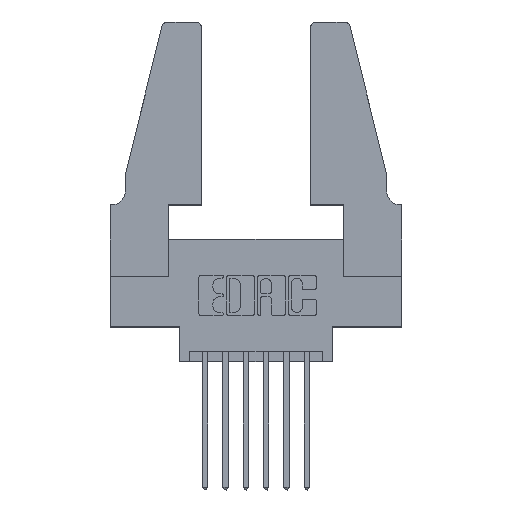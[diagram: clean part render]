
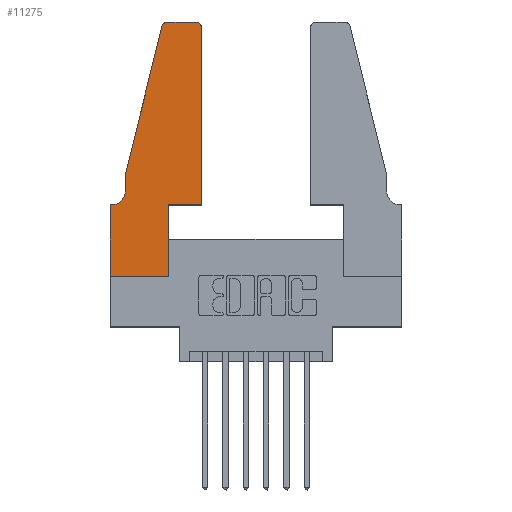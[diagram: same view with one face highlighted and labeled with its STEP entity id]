
A CAD part, top view. The second image highlights one B-rep face of the part: STEP entity #11275.
In plain terms, the highlighted planar face has unit normal (0, 0, 1).
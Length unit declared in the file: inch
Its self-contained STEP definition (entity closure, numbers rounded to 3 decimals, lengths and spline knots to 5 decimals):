
#125 = DIRECTION ( 'NONE',  ( 0., 0., 1. ) ) ;
#159 = VECTOR ( 'NONE', #10618, 39.37008 ) ;
#268 = CARTESIAN_POINT ( 'NONE',  ( 0.0755, 0.42, 0.37 ) ) ;
#296 = EDGE_CURVE ( 'NONE', #6114, #10409, #2777, .T. ) ;
#337 = ORIENTED_EDGE ( 'NONE', *, *, #775, .T. ) ;
#411 = LINE ( 'NONE', #1375, #7458 ) ;
#775 = EDGE_CURVE ( 'NONE', #4397, #8239, #9487, .T. ) ;
#880 = DIRECTION ( 'NONE',  ( 0., 1., 0. ) ) ;
#883 = AXIS2_PLACEMENT_3D ( 'NONE', #7408, #7366, #7343 ) ;
#1273 = AXIS2_PLACEMENT_3D ( 'NONE', #11120, #125, #6555 ) ;
#1285 = CARTESIAN_POINT ( 'NONE',  ( 0.4205, 1.22, 0.37 ) ) ;
#1375 = CARTESIAN_POINT ( 'NONE',  ( 0., 0., 0.37 ) ) ;
#1413 = CARTESIAN_POINT ( 'NONE',  ( 0.2865, 0., 0.37 ) ) ;
#1421 = DIRECTION ( 'NONE',  ( 1., 0., 0. ) ) ;
#1423 = DIRECTION ( 'NONE',  ( 0., 0., 1. ) ) ;
#1578 = DIRECTION ( 'NONE',  ( 0., -1., 0. ) ) ;
#1852 = VECTOR ( 'NONE', #880, 39.37008 ) ;
#2262 = CARTESIAN_POINT ( 'NONE',  ( 0.0755, 0.5, 0.37 ) ) ;
#2398 = EDGE_CURVE ( 'NONE', #9714, #2698, #7152, .T. ) ;
#2428 = ORIENTED_EDGE ( 'NONE', *, *, #6480, .T. ) ;
#2453 = AXIS2_PLACEMENT_3D ( 'NONE', #1285, #1423, #1421 ) ;
#2611 = CARTESIAN_POINT ( 'NONE',  ( 0.4505, 0.35, 0.37 ) ) ;
#2621 = LINE ( 'NONE', #8940, #8468 ) ;
#2698 = VERTEX_POINT ( 'NONE', #5643 ) ;
#2777 = LINE ( 'NONE', #4237, #4912 ) ;
#2834 = VERTEX_POINT ( 'NONE', #1413 ) ;
#2929 = LINE ( 'NONE', #4214, #159 ) ;
#2939 = ORIENTED_EDGE ( 'NONE', *, *, #296, .T. ) ;
#3159 = VERTEX_POINT ( 'NONE', #5453 ) ;
#3392 = ORIENTED_EDGE ( 'NONE', *, *, #8970, .T. ) ;
#3444 = DIRECTION ( 'NONE',  ( 1., 0., 0. ) ) ;
#3643 = EDGE_CURVE ( 'NONE', #3159, #10041, #5273, .T. ) ;
#4009 = DIRECTION ( 'NONE',  ( -0.239, -0.971, 0. ) ) ;
#4214 = CARTESIAN_POINT ( 'NONE',  ( 0., 0., 0.37 ) ) ;
#4237 = CARTESIAN_POINT ( 'NONE',  ( 0.4505, 0.35, 0.37 ) ) ;
#4397 = VERTEX_POINT ( 'NONE', #268 ) ;
#4485 = EDGE_CURVE ( 'NONE', #2834, #6114, #5528, .T. ) ;
#4746 = ORIENTED_EDGE ( 'NONE', *, *, #5229, .T. ) ;
#4912 = VECTOR ( 'NONE', #3444, 39.37008 ) ;
#5229 = EDGE_CURVE ( 'NONE', #9911, #2834, #2929, .T. ) ;
#5273 = CIRCLE ( 'NONE', #883, 0.03 ) ;
#5312 = FACE_OUTER_BOUND ( 'NONE', #9734, .T. ) ;
#5453 = CARTESIAN_POINT ( 'NONE',  ( 0.284, 1.25, 0.37 ) ) ;
#5528 = LINE ( 'NONE', #9591, #10395 ) ;
#5643 = CARTESIAN_POINT ( 'NONE',  ( 0.4205, 1.25, 0.37 ) ) ;
#5646 = PLANE ( 'NONE',  #1273 ) ;
#5889 = CARTESIAN_POINT ( 'NONE',  ( 0., 0., 0.37 ) ) ;
#5905 = LINE ( 'NONE', #9854, #10490 ) ;
#5943 = DIRECTION ( 'NONE',  ( 0., -1., 0. ) ) ;
#6023 = VECTOR ( 'NONE', #4009, 39.37008 ) ;
#6092 = CARTESIAN_POINT ( 'NONE',  ( 0.25487, 1.22718, 0.37 ) ) ;
#6114 = VERTEX_POINT ( 'NONE', #9240 ) ;
#6282 = ORIENTED_EDGE ( 'NONE', *, *, #7153, .T. ) ;
#6480 = EDGE_CURVE ( 'NONE', #8020, #4397, #5905, .T. ) ;
#6555 = DIRECTION ( 'NONE',  ( 1., 0., 0. ) ) ;
#6924 = CARTESIAN_POINT ( 'NONE',  ( 0., 0.35, 0.37 ) ) ;
#6997 = LINE ( 'NONE', #10938, #1852 ) ;
#7152 = CIRCLE ( 'NONE', #2453, 0.03 ) ;
#7153 = EDGE_CURVE ( 'NONE', #2698, #3159, #2621, .T. ) ;
#7343 = DIRECTION ( 'NONE',  ( 1., 0., 0. ) ) ;
#7366 = DIRECTION ( 'NONE',  ( 0., 0., 1. ) ) ;
#7408 = CARTESIAN_POINT ( 'NONE',  ( 0.284, 1.22, 0.37 ) ) ;
#7458 = VECTOR ( 'NONE', #5943, 39.37008 ) ;
#7779 = DIRECTION ( 'NONE',  ( 0., 1., 0. ) ) ;
#8020 = VERTEX_POINT ( 'NONE', #2262 ) ;
#8239 = VERTEX_POINT ( 'NONE', #10840 ) ;
#8261 = CARTESIAN_POINT ( 'NONE',  ( 0.0755, 0.35, 0.37 ) ) ;
#8319 = VECTOR ( 'NONE', #11016, 39.37008 ) ;
#8453 = LINE ( 'NONE', #11273, #6023 ) ;
#8468 = VECTOR ( 'NONE', #11626, 39.37008 ) ;
#8940 = CARTESIAN_POINT ( 'NONE',  ( 0.2605, 1.25, 0.37 ) ) ;
#8970 = EDGE_CURVE ( 'NONE', #10409, #9714, #6997, .T. ) ;
#9240 = CARTESIAN_POINT ( 'NONE',  ( 0.2865, 0.35, 0.37 ) ) ;
#9294 = CARTESIAN_POINT ( 'NONE',  ( 0.4505, 1.22, 0.37 ) ) ;
#9326 = AXIS2_PLACEMENT_3D ( 'NONE', #10388, #10371, #10266 ) ;
#9349 = VERTEX_POINT ( 'NONE', #6924 ) ;
#9384 = ORIENTED_EDGE ( 'NONE', *, *, #3643, .T. ) ;
#9487 = CIRCLE ( 'NONE', #9326, 0.07 ) ;
#9591 = CARTESIAN_POINT ( 'NONE',  ( 0.2865, 0.35, 0.37 ) ) ;
#9714 = VERTEX_POINT ( 'NONE', #9294 ) ;
#9734 = EDGE_LOOP ( 'NONE', ( #6282, #9384, #10839, #2428, #337, #10258, #10507, #4746, #9831, #2939, #3392, #11041 ) ) ;
#9831 = ORIENTED_EDGE ( 'NONE', *, *, #4485, .T. ) ;
#9854 = CARTESIAN_POINT ( 'NONE',  ( 0.0755, 0.5, 0.37 ) ) ;
#9911 = VERTEX_POINT ( 'NONE', #5889 ) ;
#10041 = VERTEX_POINT ( 'NONE', #6092 ) ;
#10258 = ORIENTED_EDGE ( 'NONE', *, *, #11199, .T. ) ;
#10266 = DIRECTION ( 'NONE',  ( -1., 0., 0. ) ) ;
#10371 = DIRECTION ( 'NONE',  ( 0., 0., -1. ) ) ;
#10388 = CARTESIAN_POINT ( 'NONE',  ( 0.0055, 0.42, 0.37 ) ) ;
#10395 = VECTOR ( 'NONE', #7779, 39.37008 ) ;
#10409 = VERTEX_POINT ( 'NONE', #2611 ) ;
#10490 = VECTOR ( 'NONE', #1578, 39.37008 ) ;
#10507 = ORIENTED_EDGE ( 'NONE', *, *, #10846, .T. ) ;
#10618 = DIRECTION ( 'NONE',  ( 1., 0., 0. ) ) ;
#10743 = LINE ( 'NONE', #8261, #8319 ) ;
#10839 = ORIENTED_EDGE ( 'NONE', *, *, #11414, .T. ) ;
#10840 = CARTESIAN_POINT ( 'NONE',  ( 0.0055, 0.35, 0.37 ) ) ;
#10846 = EDGE_CURVE ( 'NONE', #9349, #9911, #411, .T. ) ;
#10938 = CARTESIAN_POINT ( 'NONE',  ( 0.4505, 0.35, 0.37 ) ) ;
#11016 = DIRECTION ( 'NONE',  ( -1., 0., 0. ) ) ;
#11041 = ORIENTED_EDGE ( 'NONE', *, *, #2398, .T. ) ;
#11120 = CARTESIAN_POINT ( 'NONE',  ( 0., 0.35, 0.37 ) ) ;
#11199 = EDGE_CURVE ( 'NONE', #8239, #9349, #10743, .T. ) ;
#11273 = CARTESIAN_POINT ( 'NONE',  ( 0.0755, 0.5, 0.37 ) ) ;
#11275 = ADVANCED_FACE ( 'NONE', ( #5312 ), #5646, .T. ) ;
#11414 = EDGE_CURVE ( 'NONE', #10041, #8020, #8453, .T. ) ;
#11626 = DIRECTION ( 'NONE',  ( -1., 0., 0. ) ) ;
